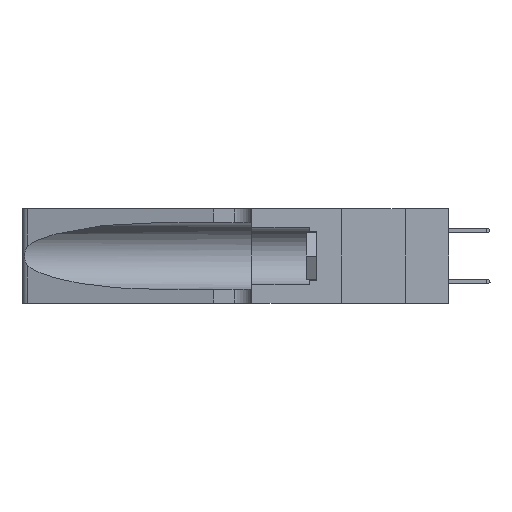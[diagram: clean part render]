
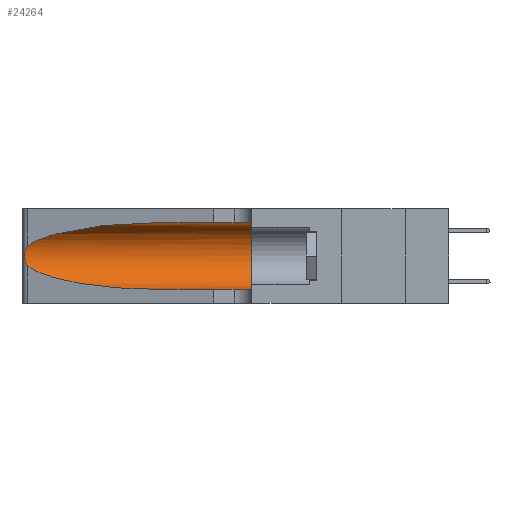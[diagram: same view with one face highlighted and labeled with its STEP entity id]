
A CAD part, left-side view. The second image highlights one B-rep face of the part: STEP entity #24264.
In plain terms, the highlighted cylindrical face has radius 3.308 mm (diameter 6.617 mm), a partial arc.
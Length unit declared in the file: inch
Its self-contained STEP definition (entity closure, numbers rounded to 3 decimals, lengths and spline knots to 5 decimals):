
#250 = VERTEX_POINT ( 'NONE', #26454 ) ;
#527 = DIRECTION ( 'NONE',  ( 0., -1., 0. ) ) ;
#943 = CARTESIAN_POINT ( 'NONE',  ( 0.26075, 1.23896, 0.178 ) ) ;
#1124 = CARTESIAN_POINT ( 'NONE',  ( 0.25487, 1.22718, 0.22369 ) ) ;
#1147 = CARTESIAN_POINT ( 'NONE',  ( 0.25487, 1.22718, 0.14631 ) ) ;
#1317 = CARTESIAN_POINT ( 'NONE',  ( 0.18966, 0.96281, 0.31525 ) ) ;
#1344 = DIRECTION ( 'NONE',  ( 0., -1., 0. ) ) ;
#1798 = DIRECTION ( 'NONE',  ( 0., 0., -1. ) ) ;
#4970 = VECTOR ( 'NONE', #527, 39.37008 ) ;
#5034 = CYLINDRICAL_SURFACE ( 'NONE', #27294, 0.13025 ) ;
#5459 = EDGE_CURVE ( 'NONE', #19481, #9126, #13244, .T. ) ;
#6197 = CARTESIAN_POINT ( 'NONE',  ( 0.1305, 0.35, 0.31525 ) ) ;
#7194 = CARTESIAN_POINT ( 'NONE',  ( 0.25639, 1.23184, 0.21858 ) ) ;
#7418 = CARTESIAN_POINT ( 'NONE',  ( 0.25487, 1.22718, 0.14631 ) ) ;
#7509 = CARTESIAN_POINT ( 'NONE',  ( 0.1305, 0.72297, 0.05475 ) ) ;
#7710 = CARTESIAN_POINT ( 'NONE',  ( 0.2373, 1.15595, 0.08982 ) ) ;
#8362 = CARTESIAN_POINT ( 'NONE',  ( 0.1305, 0.35, 0.185 ) ) ;
#8735 = EDGE_CURVE ( 'NONE', #27186, #10436, #28378, .T. ) ;
#9069 = CARTESIAN_POINT ( 'NONE',  ( 0.25555, 1.22994, 0.2215 ) ) ;
#9126 = VERTEX_POINT ( 'NONE', #21198 ) ;
#10436 = VERTEX_POINT ( 'NONE', #11400 ) ;
#10577 = DIRECTION ( 'NONE',  ( 0., -1., 0. ) ) ;
#11015 = VERTEX_POINT ( 'NONE', #12857 ) ;
#11400 = CARTESIAN_POINT ( 'NONE',  ( 0.1305, 0.35, 0.05475 ) ) ;
#11818 = EDGE_CURVE ( 'NONE', #11015, #19481, #17874, .T. ) ;
#11820 = CARTESIAN_POINT ( 'NONE',  ( 0.18966, 0.96281, 0.05475 ) ) ;
#11973 = CARTESIAN_POINT ( 'NONE',  ( 0.26018, 1.23835, 0.19895 ) ) ;
#12056 = ORIENTED_EDGE ( 'NONE', *, *, #11818, .T. ) ;
#12261 = CARTESIAN_POINT ( 'NONE',  ( 0.25639, 1.23186, 0.15144 ) ) ;
#12275 = CARTESIAN_POINT ( 'NONE',  ( 0.1305, 1.61858, 0.31525 ) ) ;
#12857 = CARTESIAN_POINT ( 'NONE',  ( 0.25487, 1.22718, 0.22369 ) ) ;
#13244 =( BOUNDED_CURVE ( )  B_SPLINE_CURVE ( 3, ( #25287, #7710, #11820, #7509 ),
 .UNSPECIFIED., .F., .F. ) 
 B_SPLINE_CURVE_WITH_KNOTS ( ( 4, 4 ),
 ( 3.44316, 4.71239 ),
 .UNSPECIFIED. ) 
 CURVE ( )  GEOMETRIC_REPRESENTATION_ITEM ( )  RATIONAL_B_SPLINE_CURVE ( ( 1., 0.87, 0.87, 1. ) ) 
 REPRESENTATION_ITEM ( '' )  );
#13586 = CARTESIAN_POINT ( 'NONE',  ( 0.25854, 1.2359, 0.20912 ) ) ;
#14115 = ORIENTED_EDGE ( 'NONE', *, *, #19034, .F. ) ;
#14261 = CARTESIAN_POINT ( 'NONE',  ( 0.26075, 1.23896, 0.19203 ) ) ;
#14836 =( BOUNDED_CURVE ( )  B_SPLINE_CURVE ( 3, ( #18802, #1317, #28160, #1124 ),
 .UNSPECIFIED., .F., .F. ) 
 B_SPLINE_CURVE_WITH_KNOTS ( ( 4, 4 ),
 ( 1.5708, 2.84003 ),
 .UNSPECIFIED. ) 
 CURVE ( )  GEOMETRIC_REPRESENTATION_ITEM ( )  RATIONAL_B_SPLINE_CURVE ( ( 1., 0.87, 0.87, 1. ) ) 
 REPRESENTATION_ITEM ( '' )  );
#15010 = LINE ( 'NONE', #12275, #22017 ) ;
#16379 = EDGE_LOOP ( 'NONE', ( #19289, #12056, #19156, #19290, #26563, #14115 ) ) ;
#16571 = CARTESIAN_POINT ( 'NONE',  ( 0.25856, 1.23593, 0.16098 ) ) ;
#16836 = FACE_OUTER_BOUND ( 'NONE', #16379, .T. ) ;
#17416 = CARTESIAN_POINT ( 'NONE',  ( 0.1305, 1.61858, 0.185 ) ) ;
#17463 = LINE ( 'NONE', #22823, #4970 ) ;
#17874 = B_SPLINE_CURVE_WITH_KNOTS ( 'NONE', 3,
 ( #20100, #9069, #7194, #27185, #13586, #11973, #14261, #943, #25440, #16571, #27382, #12261, #18921, #1147 ),
 .UNSPECIFIED., .F., .F.,
 ( 4, 2, 2, 2, 2, 2, 4 ),
 ( 0., 0.00027, 0.00053, 0.00107, 0.0016, 0.00187, 0.00214 ),
 .UNSPECIFIED. ) ;
#18802 = CARTESIAN_POINT ( 'NONE',  ( 0.1305, 0.72297, 0.31525 ) ) ;
#18921 = CARTESIAN_POINT ( 'NONE',  ( 0.25555, 1.22993, 0.14849 ) ) ;
#19034 = EDGE_CURVE ( 'NONE', #250, #27186, #15010, .T. ) ;
#19156 = ORIENTED_EDGE ( 'NONE', *, *, #5459, .T. ) ;
#19196 = DIRECTION ( 'NONE',  ( 0., 0., 1. ) ) ;
#19289 = ORIENTED_EDGE ( 'NONE', *, *, #24093, .T. ) ;
#19290 = ORIENTED_EDGE ( 'NONE', *, *, #28770, .T. ) ;
#19481 = VERTEX_POINT ( 'NONE', #7418 ) ;
#20100 = CARTESIAN_POINT ( 'NONE',  ( 0.25487, 1.22718, 0.22369 ) ) ;
#21198 = CARTESIAN_POINT ( 'NONE',  ( 0.1305, 0.72297, 0.05475 ) ) ;
#22017 = VECTOR ( 'NONE', #1344, 39.37008 ) ;
#22823 = CARTESIAN_POINT ( 'NONE',  ( 0.1305, 1.61858, 0.05475 ) ) ;
#24093 = EDGE_CURVE ( 'NONE', #250, #11015, #14836, .T. ) ;
#24264 = ADVANCED_FACE ( 'NONE', ( #16836 ), #5034, .F. ) ;
#25022 = AXIS2_PLACEMENT_3D ( 'NONE', #8362, #26017, #19196 ) ;
#25287 = CARTESIAN_POINT ( 'NONE',  ( 0.25487, 1.22718, 0.14631 ) ) ;
#25440 = CARTESIAN_POINT ( 'NONE',  ( 0.26017, 1.23833, 0.17102 ) ) ;
#26017 = DIRECTION ( 'NONE',  ( 0., 1., 0. ) ) ;
#26454 = CARTESIAN_POINT ( 'NONE',  ( 0.1305, 0.72297, 0.31525 ) ) ;
#26563 = ORIENTED_EDGE ( 'NONE', *, *, #8735, .F. ) ;
#27185 = CARTESIAN_POINT ( 'NONE',  ( 0.25787, 1.23484, 0.2124 ) ) ;
#27186 = VERTEX_POINT ( 'NONE', #6197 ) ;
#27294 = AXIS2_PLACEMENT_3D ( 'NONE', #17416, #10577, #1798 ) ;
#27382 = CARTESIAN_POINT ( 'NONE',  ( 0.25789, 1.23486, 0.15765 ) ) ;
#28160 = CARTESIAN_POINT ( 'NONE',  ( 0.2373, 1.15595, 0.28018 ) ) ;
#28378 = CIRCLE ( 'NONE', #25022, 0.13025 ) ;
#28770 = EDGE_CURVE ( 'NONE', #9126, #10436, #17463, .T. ) ;
